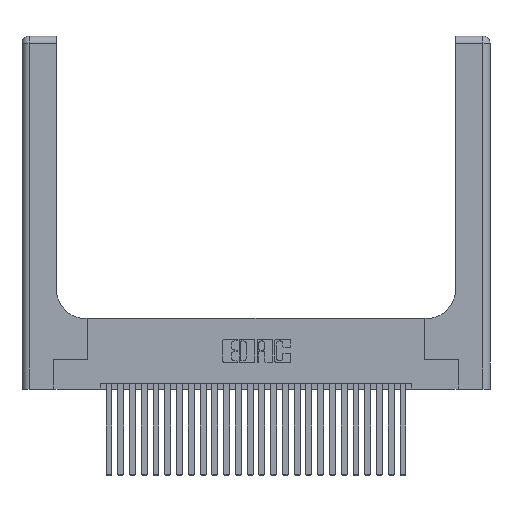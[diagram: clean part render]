
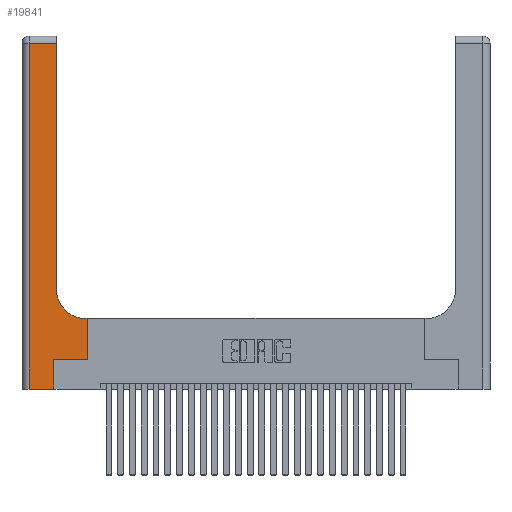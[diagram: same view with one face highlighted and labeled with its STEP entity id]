
A CAD part, top view. The second image highlights one B-rep face of the part: STEP entity #19841.
In plain terms, the highlighted planar face has unit normal (0, 0, 1).
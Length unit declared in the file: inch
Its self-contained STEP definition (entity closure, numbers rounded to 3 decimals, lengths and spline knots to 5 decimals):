
#335 = DIRECTION ( 'NONE',  ( 0., 1., 0. ) ) ;
#353 = CARTESIAN_POINT ( 'NONE',  ( 0.5585, 0.25, 0.37 ) ) ;
#1617 = DIRECTION ( 'NONE',  ( 0., 0., -1. ) ) ;
#1848 = LINE ( 'NONE', #353, #12633 ) ;
#2047 = DIRECTION ( 'NONE',  ( 1., 0., 0. ) ) ;
#2100 = EDGE_CURVE ( 'NONE', #20257, #21157, #25312, .T. ) ;
#2154 = EDGE_CURVE ( 'NONE', #23173, #20257, #12771, .T. ) ;
#2179 = VECTOR ( 'NONE', #22295, 39.37008 ) ;
#2550 = DIRECTION ( 'NONE',  ( -1., 0., 0. ) ) ;
#3246 = EDGE_CURVE ( 'NONE', #24463, #23173, #9372, .T. ) ;
#3833 = EDGE_LOOP ( 'NONE', ( #25951, #9753, #16091, #22323, #14409, #26283, #15764, #27567, #6386 ) ) ;
#4191 = CARTESIAN_POINT ( 'NONE',  ( 0.06, 3., 0.37 ) ) ;
#4366 = DIRECTION ( 'NONE',  ( 1., 0., 0. ) ) ;
#5320 = CARTESIAN_POINT ( 'NONE',  ( 0., 3., 0.37 ) ) ;
#6386 = ORIENTED_EDGE ( 'NONE', *, *, #3246, .T. ) ;
#6497 = FACE_OUTER_BOUND ( 'NONE', #3833, .T. ) ;
#7479 = CARTESIAN_POINT ( 'NONE',  ( 0.269, 0.25, 0.37 ) ) ;
#7931 = LINE ( 'NONE', #9627, #2179 ) ;
#9265 = VECTOR ( 'NONE', #2550, 39.37008 ) ;
#9372 = CIRCLE ( 'NONE', #13086, 0.25 ) ;
#9624 = AXIS2_PLACEMENT_3D ( 'NONE', #5320, #22318, #9651 ) ;
#9627 = CARTESIAN_POINT ( 'NONE',  ( 0.269, 0., 0.37 ) ) ;
#9651 = DIRECTION ( 'NONE',  ( -1., 0., 0. ) ) ;
#9753 = ORIENTED_EDGE ( 'NONE', *, *, #2100, .T. ) ;
#10149 = CARTESIAN_POINT ( 'NONE',  ( 0.06, 2.94, 0.37 ) ) ;
#10440 = CARTESIAN_POINT ( 'NONE',  ( 0.5585, 0.25, 0.37 ) ) ;
#10604 = VERTEX_POINT ( 'NONE', #22092 ) ;
#10861 = CARTESIAN_POINT ( 'NONE',  ( 0.06, 0., 0.37 ) ) ;
#11437 = VECTOR ( 'NONE', #2047, 39.37008 ) ;
#11885 = CARTESIAN_POINT ( 'NONE',  ( 0.5585, 0.6, 0.37 ) ) ;
#12355 = EDGE_CURVE ( 'NONE', #13313, #23000, #17758, .T. ) ;
#12633 = VECTOR ( 'NONE', #21677, 39.37008 ) ;
#12771 = LINE ( 'NONE', #19597, #23346 ) ;
#13086 = AXIS2_PLACEMENT_3D ( 'NONE', #14486, #1617, #16653 ) ;
#13156 = DIRECTION ( 'NONE',  ( -1., 0., 0. ) ) ;
#13313 = VERTEX_POINT ( 'NONE', #7479 ) ;
#13646 = EDGE_CURVE ( 'NONE', #20217, #10604, #25902, .T. ) ;
#14249 = LINE ( 'NONE', #17546, #9265 ) ;
#14407 = VECTOR ( 'NONE', #19155, 39.37008 ) ;
#14409 = ORIENTED_EDGE ( 'NONE', *, *, #24011, .T. ) ;
#14486 = CARTESIAN_POINT ( 'NONE',  ( 0.5415, 0.85, 0.37 ) ) ;
#15026 = CARTESIAN_POINT ( 'NONE',  ( 0., 0., 0.37 ) ) ;
#15764 = ORIENTED_EDGE ( 'NONE', *, *, #23799, .T. ) ;
#16091 = ORIENTED_EDGE ( 'NONE', *, *, #21818, .T. ) ;
#16653 = DIRECTION ( 'NONE',  ( 1., 0., 0. ) ) ;
#17357 = CARTESIAN_POINT ( 'NONE',  ( 0.2915, 2.94, 0.37 ) ) ;
#17546 = CARTESIAN_POINT ( 'NONE',  ( 0.2915, 0.6, 0.37 ) ) ;
#17758 = LINE ( 'NONE', #27491, #11437 ) ;
#19155 = DIRECTION ( 'NONE',  ( 0., -1., 0. ) ) ;
#19461 = CARTESIAN_POINT ( 'NONE',  ( 0.2915, 0.85, 0.37 ) ) ;
#19597 = CARTESIAN_POINT ( 'NONE',  ( 0.2915, 3., 0.37 ) ) ;
#19704 = VECTOR ( 'NONE', #4366, 39.37008 ) ;
#19841 = ADVANCED_FACE ( 'NONE', ( #6497 ), #20252, .F. ) ;
#19897 = VERTEX_POINT ( 'NONE', #11885 ) ;
#20217 = VERTEX_POINT ( 'NONE', #10861 ) ;
#20252 = PLANE ( 'NONE',  #9624 ) ;
#20257 = VERTEX_POINT ( 'NONE', #17357 ) ;
#20419 = VECTOR ( 'NONE', #13156, 39.37008 ) ;
#21157 = VERTEX_POINT ( 'NONE', #10149 ) ;
#21677 = DIRECTION ( 'NONE',  ( 0., 1., 0. ) ) ;
#21818 = EDGE_CURVE ( 'NONE', #21157, #20217, #24973, .T. ) ;
#22092 = CARTESIAN_POINT ( 'NONE',  ( 0.269, 0., 0.37 ) ) ;
#22295 = DIRECTION ( 'NONE',  ( 0., 1., 0. ) ) ;
#22318 = DIRECTION ( 'NONE',  ( 0., 0., -1. ) ) ;
#22323 = ORIENTED_EDGE ( 'NONE', *, *, #13646, .T. ) ;
#23000 = VERTEX_POINT ( 'NONE', #10440 ) ;
#23173 = VERTEX_POINT ( 'NONE', #19461 ) ;
#23346 = VECTOR ( 'NONE', #335, 39.37008 ) ;
#23787 = CARTESIAN_POINT ( 'NONE',  ( 0.5415, 0.6, 0.37 ) ) ;
#23799 = EDGE_CURVE ( 'NONE', #23000, #19897, #1848, .T. ) ;
#24011 = EDGE_CURVE ( 'NONE', #10604, #13313, #7931, .T. ) ;
#24463 = VERTEX_POINT ( 'NONE', #23787 ) ;
#24474 = EDGE_CURVE ( 'NONE', #19897, #24463, #14249, .T. ) ;
#24973 = LINE ( 'NONE', #4191, #14407 ) ;
#25312 = LINE ( 'NONE', #25793, #20419 ) ;
#25793 = CARTESIAN_POINT ( 'NONE',  ( 0., 2.94, 0.37 ) ) ;
#25902 = LINE ( 'NONE', #15026, #19704 ) ;
#25951 = ORIENTED_EDGE ( 'NONE', *, *, #2154, .T. ) ;
#26283 = ORIENTED_EDGE ( 'NONE', *, *, #12355, .T. ) ;
#27491 = CARTESIAN_POINT ( 'NONE',  ( 0.269, 0.25, 0.37 ) ) ;
#27567 = ORIENTED_EDGE ( 'NONE', *, *, #24474, .T. ) ;
